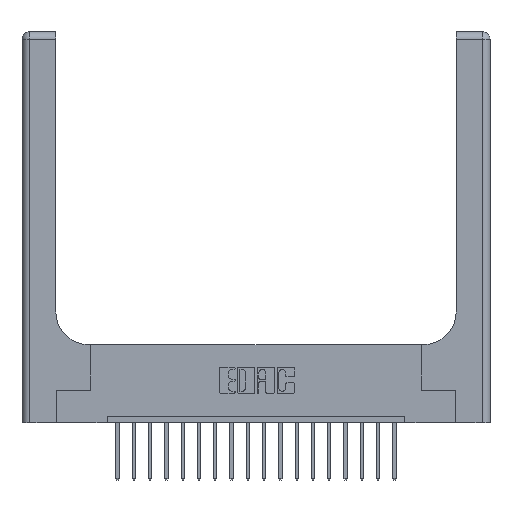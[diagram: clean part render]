
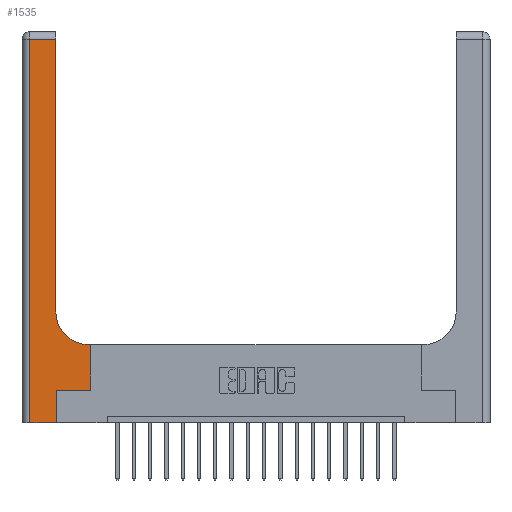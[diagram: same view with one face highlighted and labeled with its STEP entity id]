
A CAD part, top view. The second image highlights one B-rep face of the part: STEP entity #1535.
In plain terms, the highlighted planar face has unit normal (0, 0, 1).
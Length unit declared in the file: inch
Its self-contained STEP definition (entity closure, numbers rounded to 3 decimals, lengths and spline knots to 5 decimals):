
#100 = DIRECTION ( 'NONE',  ( 1., 0., 0. ) ) ;
#187 = CARTESIAN_POINT ( 'NONE',  ( 0.265, 0., 0.37 ) ) ;
#377 = VECTOR ( 'NONE', #8025, 39.37008 ) ;
#907 = LINE ( 'NONE', #11157, #10148 ) ;
#993 = ORIENTED_EDGE ( 'NONE', *, *, #10762, .T. ) ;
#1161 = EDGE_CURVE ( 'NONE', #8308, #3571, #11637, .T. ) ;
#1397 = VECTOR ( 'NONE', #17906, 39.37008 ) ;
#1402 = VERTEX_POINT ( 'NONE', #11935 ) ;
#1417 = VERTEX_POINT ( 'NONE', #16375 ) ;
#1531 = VERTEX_POINT ( 'NONE', #10843 ) ;
#1535 = ADVANCED_FACE ( 'NONE', ( #15430 ), #18319, .F. ) ;
#1543 = DIRECTION ( 'NONE',  ( -1., 0., 0. ) ) ;
#2723 = CARTESIAN_POINT ( 'NONE',  ( 0.528, 0.6, 0.37 ) ) ;
#3061 = CARTESIAN_POINT ( 'NONE',  ( 0.528, 0.25, 0.37 ) ) ;
#3270 = DIRECTION ( 'NONE',  ( 0., 0., -1. ) ) ;
#3571 = VERTEX_POINT ( 'NONE', #5094 ) ;
#3743 = ORIENTED_EDGE ( 'NONE', *, *, #1161, .T. ) ;
#4646 = ORIENTED_EDGE ( 'NONE', *, *, #18883, .T. ) ;
#4701 = CARTESIAN_POINT ( 'NONE',  ( 0.51, 0.85, 0.37 ) ) ;
#4729 = LINE ( 'NONE', #4894, #4931 ) ;
#4894 = CARTESIAN_POINT ( 'NONE',  ( 0.26, 3., 0.37 ) ) ;
#4931 = VECTOR ( 'NONE', #10927, 39.37008 ) ;
#5094 = CARTESIAN_POINT ( 'NONE',  ( 0.265, 0.25, 0.37 ) ) ;
#5294 = LINE ( 'NONE', #6527, #377 ) ;
#5553 = EDGE_CURVE ( 'NONE', #3571, #12761, #9104, .T. ) ;
#5644 = CARTESIAN_POINT ( 'NONE',  ( 0.265, 0.25, 0.37 ) ) ;
#5913 = AXIS2_PLACEMENT_3D ( 'NONE', #18266, #9254, #1543 ) ;
#5950 = VERTEX_POINT ( 'NONE', #9432 ) ;
#6527 = CARTESIAN_POINT ( 'NONE',  ( 0., 0., 0.37 ) ) ;
#7501 = VERTEX_POINT ( 'NONE', #17340 ) ;
#8025 = DIRECTION ( 'NONE',  ( 1., 0., 0. ) ) ;
#8308 = VERTEX_POINT ( 'NONE', #187 ) ;
#8493 = LINE ( 'NONE', #16291, #1397 ) ;
#8997 = ORIENTED_EDGE ( 'NONE', *, *, #5553, .T. ) ;
#9104 = LINE ( 'NONE', #5644, #15788 ) ;
#9229 = DIRECTION ( 'NONE',  ( 0., 1., 0. ) ) ;
#9254 = DIRECTION ( 'NONE',  ( 0., 0., -1. ) ) ;
#9432 = CARTESIAN_POINT ( 'NONE',  ( 0.26, 2.94, 0.37 ) ) ;
#10148 = VECTOR ( 'NONE', #17397, 39.37008 ) ;
#10183 = EDGE_CURVE ( 'NONE', #10662, #1531, #14435, .T. ) ;
#10662 = VERTEX_POINT ( 'NONE', #2723 ) ;
#10672 = DIRECTION ( 'NONE',  ( -1., 0., 0. ) ) ;
#10762 = EDGE_CURVE ( 'NONE', #12761, #10662, #18369, .T. ) ;
#10797 = ORIENTED_EDGE ( 'NONE', *, *, #17497, .T. ) ;
#10843 = CARTESIAN_POINT ( 'NONE',  ( 0.51, 0.6, 0.37 ) ) ;
#10927 = DIRECTION ( 'NONE',  ( 0., 1., 0. ) ) ;
#11157 = CARTESIAN_POINT ( 'NONE',  ( 0.06, 3., 0.37 ) ) ;
#11192 = AXIS2_PLACEMENT_3D ( 'NONE', #4701, #3270, #100 ) ;
#11199 = ORIENTED_EDGE ( 'NONE', *, *, #10183, .T. ) ;
#11637 = LINE ( 'NONE', #15344, #14532 ) ;
#11784 = EDGE_CURVE ( 'NONE', #1402, #5950, #4729, .T. ) ;
#11935 = CARTESIAN_POINT ( 'NONE',  ( 0.26, 0.85, 0.37 ) ) ;
#12382 = ORIENTED_EDGE ( 'NONE', *, *, #16443, .T. ) ;
#12761 = VERTEX_POINT ( 'NONE', #16905 ) ;
#12860 = EDGE_CURVE ( 'NONE', #1417, #8308, #5294, .T. ) ;
#13183 = DIRECTION ( 'NONE',  ( 1., 0., 0. ) ) ;
#14184 = VECTOR ( 'NONE', #10672, 39.37008 ) ;
#14435 = LINE ( 'NONE', #18230, #14184 ) ;
#14532 = VECTOR ( 'NONE', #9229, 39.37008 ) ;
#15258 = DIRECTION ( 'NONE',  ( 0., 1., 0. ) ) ;
#15344 = CARTESIAN_POINT ( 'NONE',  ( 0.265, 0., 0.37 ) ) ;
#15430 = FACE_OUTER_BOUND ( 'NONE', #18751, .T. ) ;
#15788 = VECTOR ( 'NONE', #13183, 39.37008 ) ;
#16291 = CARTESIAN_POINT ( 'NONE',  ( 0., 2.94, 0.37 ) ) ;
#16375 = CARTESIAN_POINT ( 'NONE',  ( 0.06, 0., 0.37 ) ) ;
#16443 = EDGE_CURVE ( 'NONE', #5950, #7501, #8493, .T. ) ;
#16905 = CARTESIAN_POINT ( 'NONE',  ( 0.528, 0.25, 0.37 ) ) ;
#16953 = ORIENTED_EDGE ( 'NONE', *, *, #11784, .T. ) ;
#17233 = VECTOR ( 'NONE', #15258, 39.37008 ) ;
#17340 = CARTESIAN_POINT ( 'NONE',  ( 0.06, 2.94, 0.37 ) ) ;
#17397 = DIRECTION ( 'NONE',  ( 0., -1., 0. ) ) ;
#17497 = EDGE_CURVE ( 'NONE', #7501, #1417, #907, .T. ) ;
#17906 = DIRECTION ( 'NONE',  ( -1., 0., 0. ) ) ;
#18230 = CARTESIAN_POINT ( 'NONE',  ( 0.26, 0.6, 0.37 ) ) ;
#18266 = CARTESIAN_POINT ( 'NONE',  ( 0., 3., 0.37 ) ) ;
#18319 = PLANE ( 'NONE',  #5913 ) ;
#18369 = LINE ( 'NONE', #3061, #17233 ) ;
#18402 = ORIENTED_EDGE ( 'NONE', *, *, #12860, .T. ) ;
#18557 = CIRCLE ( 'NONE', #11192, 0.25 ) ;
#18751 = EDGE_LOOP ( 'NONE', ( #16953, #12382, #10797, #18402, #3743, #8997, #993, #11199, #4646 ) ) ;
#18883 = EDGE_CURVE ( 'NONE', #1531, #1402, #18557, .T. ) ;
